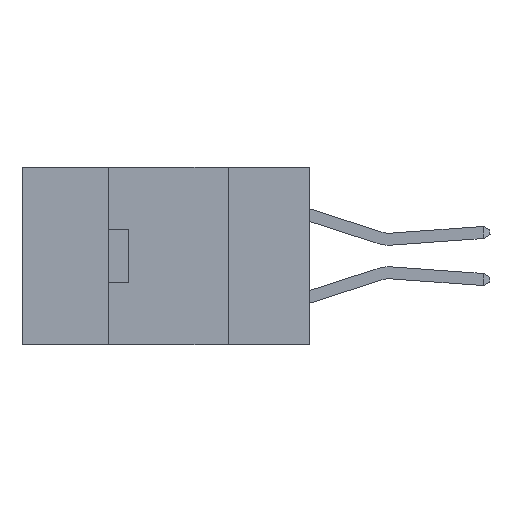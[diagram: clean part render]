
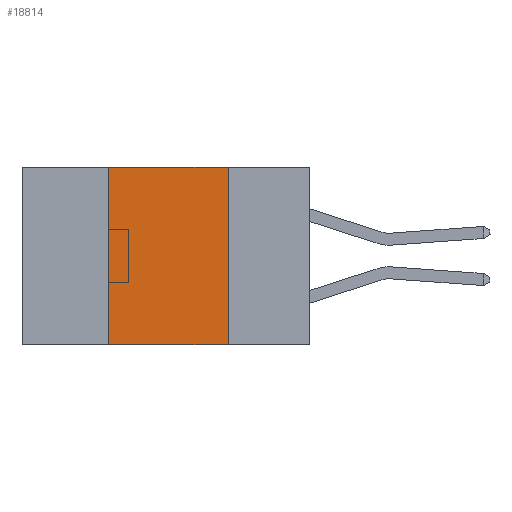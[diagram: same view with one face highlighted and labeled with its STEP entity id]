
A CAD part, left-side view. The second image highlights one B-rep face of the part: STEP entity #18814.
In plain terms, the highlighted planar face has unit normal (-1, 0, 0).
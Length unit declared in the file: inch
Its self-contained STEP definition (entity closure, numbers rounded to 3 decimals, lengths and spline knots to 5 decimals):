
#963 = EDGE_CURVE ( 'NONE', #22447, #2281, #15337, .T. ) ;
#1685 = AXIS2_PLACEMENT_3D ( 'NONE', #5468, #20597, #7685 ) ;
#1751 = LINE ( 'NONE', #6497, #6931 ) ;
#2103 = LINE ( 'NONE', #16702, #6603 ) ;
#2281 = VERTEX_POINT ( 'NONE', #23819 ) ;
#5056 = ORIENTED_EDGE ( 'NONE', *, *, #8157, .T. ) ;
#5468 = CARTESIAN_POINT ( 'NONE',  ( 0., 0.6, 0. ) ) ;
#6080 = DIRECTION ( 'NONE',  ( 0., 0., -1. ) ) ;
#6399 = FACE_OUTER_BOUND ( 'NONE', #22950, .T. ) ;
#6497 = CARTESIAN_POINT ( 'NONE',  ( 0., 0.6, -0.37 ) ) ;
#6603 = VECTOR ( 'NONE', #12389, 39.37008 ) ;
#6931 = VECTOR ( 'NONE', #21568, 39.37008 ) ;
#7195 = VERTEX_POINT ( 'NONE', #16846 ) ;
#7685 = DIRECTION ( 'NONE',  ( 0., 0., -1. ) ) ;
#7964 = EDGE_CURVE ( 'NONE', #7195, #22447, #2103, .T. ) ;
#8157 = EDGE_CURVE ( 'NONE', #7195, #27836, #1751, .T. ) ;
#9491 = ORIENTED_EDGE ( 'NONE', *, *, #963, .F. ) ;
#11429 = CARTESIAN_POINT ( 'NONE',  ( 0., 0.6, 0. ) ) ;
#12389 = DIRECTION ( 'NONE',  ( 0., 0., 1. ) ) ;
#14579 = ORIENTED_EDGE ( 'NONE', *, *, #20312, .F. ) ;
#15337 = LINE ( 'NONE', #11429, #21030 ) ;
#16702 = CARTESIAN_POINT ( 'NONE',  ( 0., 0.42, -0.37 ) ) ;
#16846 = CARTESIAN_POINT ( 'NONE',  ( 0., 0.42, -0.37 ) ) ;
#18425 = PLANE ( 'NONE',  #1685 ) ;
#18814 = ADVANCED_FACE ( 'NONE', ( #6399 ), #18425, .F. ) ;
#19016 = CARTESIAN_POINT ( 'NONE',  ( 0., 0.17, -0.37 ) ) ;
#20312 = EDGE_CURVE ( 'NONE', #2281, #27836, #25111, .T. ) ;
#20597 = DIRECTION ( 'NONE',  ( 1., 0., 0. ) ) ;
#20955 = ORIENTED_EDGE ( 'NONE', *, *, #7964, .F. ) ;
#21030 = VECTOR ( 'NONE', #26378, 39.37008 ) ;
#21360 = CARTESIAN_POINT ( 'NONE',  ( 0., 0.17, -0.37 ) ) ;
#21568 = DIRECTION ( 'NONE',  ( 0., -1., 0. ) ) ;
#22447 = VERTEX_POINT ( 'NONE', #23858 ) ;
#22950 = EDGE_LOOP ( 'NONE', ( #14579, #9491, #20955, #5056 ) ) ;
#23819 = CARTESIAN_POINT ( 'NONE',  ( 0., 0.17, 0. ) ) ;
#23858 = CARTESIAN_POINT ( 'NONE',  ( 0., 0.42, 0. ) ) ;
#24453 = VECTOR ( 'NONE', #6080, 39.37008 ) ;
#25111 = LINE ( 'NONE', #19016, #24453 ) ;
#26378 = DIRECTION ( 'NONE',  ( 0., -1., 0. ) ) ;
#27836 = VERTEX_POINT ( 'NONE', #21360 ) ;
